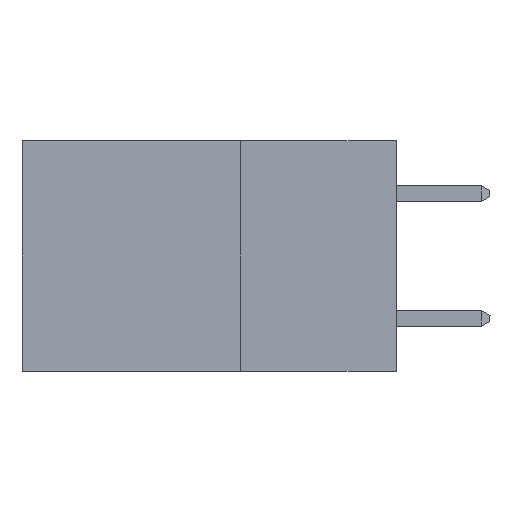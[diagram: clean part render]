
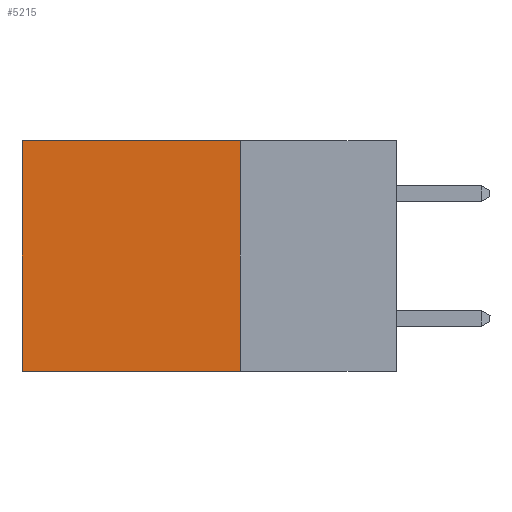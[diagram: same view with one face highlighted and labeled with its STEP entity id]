
A CAD part, left-side view. The second image highlights one B-rep face of the part: STEP entity #5215.
In plain terms, the highlighted planar face has unit normal (-1, 0, 0).
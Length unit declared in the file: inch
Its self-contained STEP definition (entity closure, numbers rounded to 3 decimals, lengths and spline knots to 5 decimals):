
#225 = VECTOR ( 'NONE', #11194, 39.37008 ) ;
#415 = FACE_OUTER_BOUND ( 'NONE', #14935, .T. ) ;
#1028 = CARTESIAN_POINT ( 'NONE',  ( 0.298, 0.25, -0.37 ) ) ;
#1375 = CARTESIAN_POINT ( 'NONE',  ( 0.298, 0.25, 0. ) ) ;
#1644 = ORIENTED_EDGE ( 'NONE', *, *, #7476, .F. ) ;
#2020 = DIRECTION ( 'NONE',  ( 0., 0., -1. ) ) ;
#3107 = EDGE_CURVE ( 'NONE', #11728, #7701, #13898, .T. ) ;
#3394 = DIRECTION ( 'NONE',  ( 1., 0., 0. ) ) ;
#3760 = VECTOR ( 'NONE', #8940, 39.37008 ) ;
#3893 = CARTESIAN_POINT ( 'NONE',  ( 0.298, 0.6, 0. ) ) ;
#4285 = AXIS2_PLACEMENT_3D ( 'NONE', #4621, #3394, #2020 ) ;
#4621 = CARTESIAN_POINT ( 'NONE',  ( 0.298, 0.25, 0. ) ) ;
#5109 = CARTESIAN_POINT ( 'NONE',  ( 0.298, 0.25, -0.37 ) ) ;
#5215 = ADVANCED_FACE ( 'NONE', ( #415 ), #10754, .F. ) ;
#5337 = EDGE_CURVE ( 'NONE', #9135, #7701, #15909, .T. ) ;
#6092 = DIRECTION ( 'NONE',  ( 0., 1., 0. ) ) ;
#6750 = LINE ( 'NONE', #13836, #13941 ) ;
#6831 = ORIENTED_EDGE ( 'NONE', *, *, #7363, .T. ) ;
#7363 = EDGE_CURVE ( 'NONE', #14965, #11728, #7930, .T. ) ;
#7476 = EDGE_CURVE ( 'NONE', #14965, #9135, #6750, .T. ) ;
#7701 = VERTEX_POINT ( 'NONE', #11131 ) ;
#7930 = LINE ( 'NONE', #13708, #11948 ) ;
#8239 = CARTESIAN_POINT ( 'NONE',  ( 0.298, 0.6, 0. ) ) ;
#8472 = ORIENTED_EDGE ( 'NONE', *, *, #3107, .T. ) ;
#8940 = DIRECTION ( 'NONE',  ( 0., 0., -1. ) ) ;
#9135 = VERTEX_POINT ( 'NONE', #5109 ) ;
#10754 = PLANE ( 'NONE',  #4285 ) ;
#11131 = CARTESIAN_POINT ( 'NONE',  ( 0.298, 0.6, -0.37 ) ) ;
#11194 = DIRECTION ( 'NONE',  ( 0., 1., 0. ) ) ;
#11666 = DIRECTION ( 'NONE',  ( 0., 0., -1. ) ) ;
#11728 = VERTEX_POINT ( 'NONE', #8239 ) ;
#11948 = VECTOR ( 'NONE', #6092, 39.37008 ) ;
#12245 = ORIENTED_EDGE ( 'NONE', *, *, #5337, .F. ) ;
#13708 = CARTESIAN_POINT ( 'NONE',  ( 0.298, 0.25, 0. ) ) ;
#13836 = CARTESIAN_POINT ( 'NONE',  ( 0.298, 0.25, 0. ) ) ;
#13898 = LINE ( 'NONE', #3893, #3760 ) ;
#13941 = VECTOR ( 'NONE', #11666, 39.37008 ) ;
#14935 = EDGE_LOOP ( 'NONE', ( #8472, #12245, #1644, #6831 ) ) ;
#14965 = VERTEX_POINT ( 'NONE', #1375 ) ;
#15909 = LINE ( 'NONE', #1028, #225 ) ;
